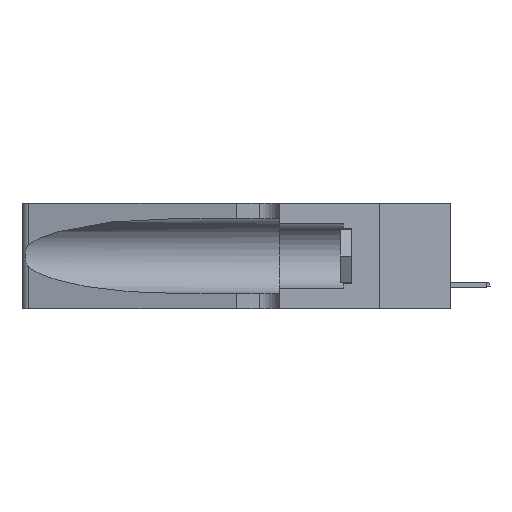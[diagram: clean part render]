
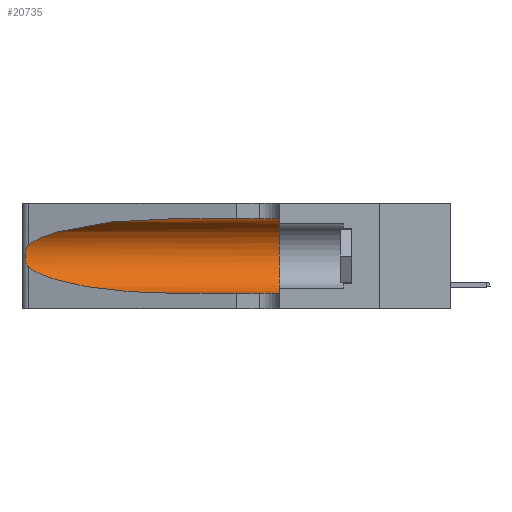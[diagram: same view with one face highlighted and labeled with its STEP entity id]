
A CAD part, left-side view. The second image highlights one B-rep face of the part: STEP entity #20735.
In plain terms, the highlighted cylindrical face has radius 3.308 mm (diameter 6.617 mm), a partial arc.
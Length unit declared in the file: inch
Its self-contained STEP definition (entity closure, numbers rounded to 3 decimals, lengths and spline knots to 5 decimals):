
#394 = ORIENTED_EDGE ( 'NONE', *, *, #6999, .T. ) ;
#505 = CARTESIAN_POINT ( 'NONE',  ( 0.2373, 1.15595, 0.08982 ) ) ;
#946 = CARTESIAN_POINT ( 'NONE',  ( 0.1305, 0.35, 0.31525 ) ) ;
#1911 = DIRECTION ( 'NONE',  ( 0., -1., 0. ) ) ;
#2348 = ORIENTED_EDGE ( 'NONE', *, *, #11281, .T. ) ;
#2371 = DIRECTION ( 'NONE',  ( 0., -1., 0. ) ) ;
#2452 = CARTESIAN_POINT ( 'NONE',  ( 0.2373, 1.15595, 0.28018 ) ) ;
#2788 = VERTEX_POINT ( 'NONE', #9248 ) ;
#2805 = DIRECTION ( 'NONE',  ( 0., 0., 1. ) ) ;
#2930 = DIRECTION ( 'NONE',  ( 0., 1., 0. ) ) ;
#3330 = EDGE_CURVE ( 'NONE', #14561, #16457, #11237, .T. ) ;
#3411 = CARTESIAN_POINT ( 'NONE',  ( 0.26075, 1.23896, 0.19203 ) ) ;
#3527 = CARTESIAN_POINT ( 'NONE',  ( 0.25639, 1.23186, 0.15144 ) ) ;
#4936 = VECTOR ( 'NONE', #21513, 39.37008 ) ;
#5630 = CARTESIAN_POINT ( 'NONE',  ( 0.18966, 0.96281, 0.05475 ) ) ;
#5664 = CARTESIAN_POINT ( 'NONE',  ( 0.25487, 1.22718, 0.14631 ) ) ;
#5678 = CIRCLE ( 'NONE', #20312, 0.13025 ) ;
#6250 = CARTESIAN_POINT ( 'NONE',  ( 0.25487, 1.22718, 0.22369 ) ) ;
#6959 = CARTESIAN_POINT ( 'NONE',  ( 0.25854, 1.2359, 0.20912 ) ) ;
#6999 = EDGE_CURVE ( 'NONE', #16457, #8300, #10059, .T. ) ;
#7522 = EDGE_LOOP ( 'NONE', ( #18268, #394, #22291, #2348, #17462, #15501 ) ) ;
#7761 = CARTESIAN_POINT ( 'NONE',  ( 0.1305, 0.72297, 0.05475 ) ) ;
#8300 = VERTEX_POINT ( 'NONE', #5664 ) ;
#8752 = CARTESIAN_POINT ( 'NONE',  ( 0.25487, 1.22718, 0.22369 ) ) ;
#9248 = CARTESIAN_POINT ( 'NONE',  ( 0.1305, 0.35, 0.05475 ) ) ;
#9708 =( BOUNDED_CURVE ( )  B_SPLINE_CURVE ( 3, ( #16698, #505, #5630, #7761 ),
 .UNSPECIFIED., .F., .T. ) 
 B_SPLINE_CURVE_WITH_KNOTS ( ( 4, 4 ),
 ( 3.44316, 4.71239 ),
 .UNSPECIFIED. ) 
 CURVE ( )  GEOMETRIC_REPRESENTATION_ITEM ( )  RATIONAL_B_SPLINE_CURVE ( ( 1., 0.87, 0.87, 1. ) ) 
 REPRESENTATION_ITEM ( '' )  );
#10059 = B_SPLINE_CURVE_WITH_KNOTS ( 'NONE', 3,
 ( #8752, #15916, #23099, #10723, #6959, #19560, #3411, #23229, #12505, #19671, #17929, #3527, #12861, #20016 ),
 .UNSPECIFIED., .F., .F.,
 ( 4, 2, 2, 2, 2, 2, 4 ),
 ( 0., 0.00027, 0.00053, 0.00107, 0.0016, 0.00187, 0.00214 ),
 .UNSPECIFIED. ) ;
#10723 = CARTESIAN_POINT ( 'NONE',  ( 0.25787, 1.23484, 0.2124 ) ) ;
#11150 = CARTESIAN_POINT ( 'NONE',  ( 0.1305, 1.61858, 0.185 ) ) ;
#11237 =( BOUNDED_CURVE ( )  B_SPLINE_CURVE ( 3, ( #15225, #20833, #2452, #6250 ),
 .UNSPECIFIED., .F., .T. ) 
 B_SPLINE_CURVE_WITH_KNOTS ( ( 4, 4 ),
 ( 1.5708, 2.84003 ),
 .UNSPECIFIED. ) 
 CURVE ( )  GEOMETRIC_REPRESENTATION_ITEM ( )  RATIONAL_B_SPLINE_CURVE ( ( 1., 0.87, 0.87, 1. ) ) 
 REPRESENTATION_ITEM ( '' )  );
#11281 = EDGE_CURVE ( 'NONE', #11817, #2788, #13276, .T. ) ;
#11376 = CARTESIAN_POINT ( 'NONE',  ( 0.1305, 1.61858, 0.05475 ) ) ;
#11611 = CARTESIAN_POINT ( 'NONE',  ( 0.1305, 0.72297, 0.05475 ) ) ;
#11817 = VERTEX_POINT ( 'NONE', #11611 ) ;
#12505 = CARTESIAN_POINT ( 'NONE',  ( 0.26017, 1.23833, 0.17102 ) ) ;
#12705 = LINE ( 'NONE', #19642, #4936 ) ;
#12861 = CARTESIAN_POINT ( 'NONE',  ( 0.25555, 1.22993, 0.14849 ) ) ;
#13185 = CARTESIAN_POINT ( 'NONE',  ( 0.1305, 0.72297, 0.31525 ) ) ;
#13276 = LINE ( 'NONE', #11376, #15668 ) ;
#14561 = VERTEX_POINT ( 'NONE', #13185 ) ;
#15225 = CARTESIAN_POINT ( 'NONE',  ( 0.1305, 0.72297, 0.31525 ) ) ;
#15501 = ORIENTED_EDGE ( 'NONE', *, *, #17635, .F. ) ;
#15535 = EDGE_CURVE ( 'NONE', #17374, #2788, #5678, .T. ) ;
#15668 = VECTOR ( 'NONE', #2371, 39.37008 ) ;
#15816 = CARTESIAN_POINT ( 'NONE',  ( 0.1305, 0.35, 0.185 ) ) ;
#15916 = CARTESIAN_POINT ( 'NONE',  ( 0.25555, 1.22994, 0.2215 ) ) ;
#16211 = FACE_OUTER_BOUND ( 'NONE', #7522, .T. ) ;
#16457 = VERTEX_POINT ( 'NONE', #17489 ) ;
#16698 = CARTESIAN_POINT ( 'NONE',  ( 0.25487, 1.22718, 0.14631 ) ) ;
#17374 = VERTEX_POINT ( 'NONE', #946 ) ;
#17462 = ORIENTED_EDGE ( 'NONE', *, *, #15535, .F. ) ;
#17489 = CARTESIAN_POINT ( 'NONE',  ( 0.25487, 1.22718, 0.22369 ) ) ;
#17635 = EDGE_CURVE ( 'NONE', #14561, #17374, #12705, .T. ) ;
#17929 = CARTESIAN_POINT ( 'NONE',  ( 0.25789, 1.23486, 0.15765 ) ) ;
#18268 = ORIENTED_EDGE ( 'NONE', *, *, #3330, .T. ) ;
#19375 = AXIS2_PLACEMENT_3D ( 'NONE', #11150, #1911, #21735 ) ;
#19560 = CARTESIAN_POINT ( 'NONE',  ( 0.26018, 1.23835, 0.19895 ) ) ;
#19642 = CARTESIAN_POINT ( 'NONE',  ( 0.1305, 1.61858, 0.31525 ) ) ;
#19671 = CARTESIAN_POINT ( 'NONE',  ( 0.25856, 1.23593, 0.16098 ) ) ;
#19853 = CYLINDRICAL_SURFACE ( 'NONE', #19375, 0.13025 ) ;
#20016 = CARTESIAN_POINT ( 'NONE',  ( 0.25487, 1.22718, 0.14631 ) ) ;
#20312 = AXIS2_PLACEMENT_3D ( 'NONE', #15816, #2930, #2805 ) ;
#20735 = ADVANCED_FACE ( 'NONE', ( #16211 ), #19853, .F. ) ;
#20833 = CARTESIAN_POINT ( 'NONE',  ( 0.18966, 0.96281, 0.31525 ) ) ;
#21513 = DIRECTION ( 'NONE',  ( 0., -1., 0. ) ) ;
#21735 = DIRECTION ( 'NONE',  ( 0., 0., -1. ) ) ;
#22291 = ORIENTED_EDGE ( 'NONE', *, *, #22978, .T. ) ;
#22978 = EDGE_CURVE ( 'NONE', #8300, #11817, #9708, .T. ) ;
#23099 = CARTESIAN_POINT ( 'NONE',  ( 0.25639, 1.23184, 0.21858 ) ) ;
#23229 = CARTESIAN_POINT ( 'NONE',  ( 0.26075, 1.23896, 0.178 ) ) ;
